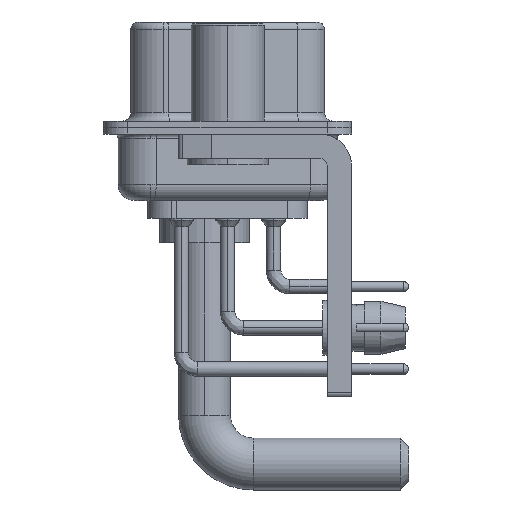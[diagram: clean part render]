
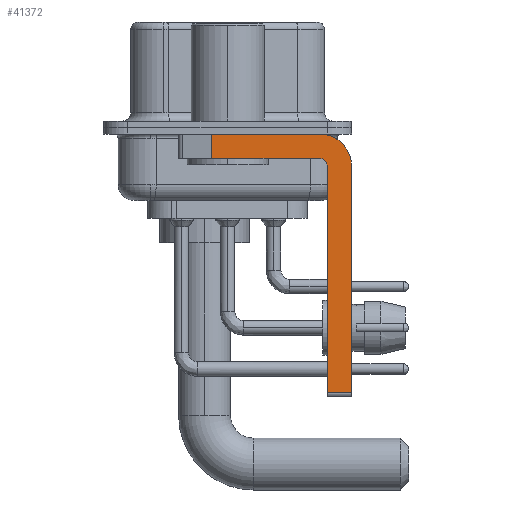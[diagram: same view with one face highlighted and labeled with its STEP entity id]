
A CAD part, left-side view. The second image highlights one B-rep face of the part: STEP entity #41372.
In plain terms, the highlighted planar face has unit normal (-1, 0, 0).
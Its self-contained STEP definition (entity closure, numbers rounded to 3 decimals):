
#185 = DIRECTION ( 'NONE',  ( 0., 0., -1. ) ) ;
#646 = CARTESIAN_POINT ( 'NONE',  ( -2.9, -7.65, -2.4 ) ) ;
#2032 = VERTEX_POINT ( 'NONE', #33714 ) ;
#2073 = LINE ( 'NONE', #14903, #31735 ) ;
#2317 = VECTOR ( 'NONE', #3384, 1000. ) ;
#2344 = EDGE_CURVE ( 'NONE', #15517, #5914, #19631, .T. ) ;
#2414 = ORIENTED_EDGE ( 'NONE', *, *, #25078, .F. ) ;
#2824 = VERTEX_POINT ( 'NONE', #13283 ) ;
#3009 = AXIS2_PLACEMENT_3D ( 'NONE', #11537, #37170, #8401 ) ;
#3141 = VERTEX_POINT ( 'NONE', #37407 ) ;
#3384 = DIRECTION ( 'NONE',  ( 0., -1., 0. ) ) ;
#4079 = DIRECTION ( 'NONE',  ( 0., 0., 1. ) ) ;
#4581 = ORIENTED_EDGE ( 'NONE', *, *, #2344, .F. ) ;
#4689 = DIRECTION ( 'NONE',  ( 0., 0., -1. ) ) ;
#5914 = VERTEX_POINT ( 'NONE', #8955 ) ;
#6447 = EDGE_CURVE ( 'NONE', #36493, #2032, #35358, .T. ) ;
#7075 = AXIS2_PLACEMENT_3D ( 'NONE', #7746, #20573, #36117 ) ;
#7746 = CARTESIAN_POINT ( 'NONE',  ( -2.9, -5.65, -2.4 ) ) ;
#7893 = AXIS2_PLACEMENT_3D ( 'NONE', #8662, #14952, #4689 ) ;
#8157 = EDGE_CURVE ( 'NONE', #36493, #9565, #31938, .T. ) ;
#8331 = ORIENTED_EDGE ( 'NONE', *, *, #39538, .T. ) ;
#8401 = DIRECTION ( 'NONE',  ( 0., 0., -1. ) ) ;
#8662 = CARTESIAN_POINT ( 'NONE',  ( -2.9, -5.65, -2.4 ) ) ;
#8955 = CARTESIAN_POINT ( 'NONE',  ( -2.9, -6.15, -2.4 ) ) ;
#9565 = VERTEX_POINT ( 'NONE', #18904 ) ;
#11042 = EDGE_CURVE ( 'NONE', #5914, #3141, #39941, .T. ) ;
#11537 = CARTESIAN_POINT ( 'NONE',  ( -2.9, -5.65, -2.4 ) ) ;
#12377 = VECTOR ( 'NONE', #185, 1000. ) ;
#13283 = CARTESIAN_POINT ( 'NONE',  ( -2.9, -7.65, -16.35 ) ) ;
#14903 = CARTESIAN_POINT ( 'NONE',  ( -2.9, -5.65, -1.9 ) ) ;
#14952 = DIRECTION ( 'NONE',  ( 1., 0., 0. ) ) ;
#15129 = PLANE ( 'NONE',  #3009 ) ;
#15517 = VERTEX_POINT ( 'NONE', #22314 ) ;
#16001 = CARTESIAN_POINT ( 'NONE',  ( -2.9, 0.978, -1.9 ) ) ;
#16626 = CIRCLE ( 'NONE', #7893, 2. ) ;
#16818 = ORIENTED_EDGE ( 'NONE', *, *, #6447, .F. ) ;
#18274 = FACE_OUTER_BOUND ( 'NONE', #23583, .T. ) ;
#18904 = CARTESIAN_POINT ( 'NONE',  ( -2.9, 0.978, -1.9 ) ) ;
#19631 = LINE ( 'NONE', #35584, #34057 ) ;
#20573 = DIRECTION ( 'NONE',  ( -1., 0., 0. ) ) ;
#21625 = DIRECTION ( 'NONE',  ( 0., 1., 0. ) ) ;
#21863 = LINE ( 'NONE', #32135, #12377 ) ;
#22314 = CARTESIAN_POINT ( 'NONE',  ( -2.9, -6.15, -16.35 ) ) ;
#22621 = ORIENTED_EDGE ( 'NONE', *, *, #8157, .T. ) ;
#23583 = EDGE_LOOP ( 'NONE', ( #16818, #22621, #32466, #31958, #4581, #8331, #2414, #29127 ) ) ;
#25078 = EDGE_CURVE ( 'NONE', #39558, #2824, #21863, .T. ) ;
#25511 = CARTESIAN_POINT ( 'NONE',  ( -2.9, 3., -0.4 ) ) ;
#28811 = DIRECTION ( 'NONE',  ( 0., 0., -1. ) ) ;
#29127 = ORIENTED_EDGE ( 'NONE', *, *, #33601, .F. ) ;
#31735 = VECTOR ( 'NONE', #21625, 1000. ) ;
#31938 = LINE ( 'NONE', #16001, #33811 ) ;
#31958 = ORIENTED_EDGE ( 'NONE', *, *, #11042, .F. ) ;
#32135 = CARTESIAN_POINT ( 'NONE',  ( -2.9, -7.65, -2.4 ) ) ;
#32466 = ORIENTED_EDGE ( 'NONE', *, *, #38532, .F. ) ;
#33601 = EDGE_CURVE ( 'NONE', #2032, #39558, #16626, .T. ) ;
#33714 = CARTESIAN_POINT ( 'NONE',  ( -2.9, -5.65, -0.4 ) ) ;
#33811 = VECTOR ( 'NONE', #28811, 1000. ) ;
#34057 = VECTOR ( 'NONE', #4079, 1000. ) ;
#34525 = DIRECTION ( 'NONE',  ( 0., -1., 0. ) ) ;
#35358 = LINE ( 'NONE', #25511, #39803 ) ;
#35389 = CARTESIAN_POINT ( 'NONE',  ( -2.9, 0.978, -0.4 ) ) ;
#35584 = CARTESIAN_POINT ( 'NONE',  ( -2.9, -6.15, -16.6 ) ) ;
#35725 = LINE ( 'NONE', #38260, #2317 ) ;
#36117 = DIRECTION ( 'NONE',  ( 0., 0., 1. ) ) ;
#36493 = VERTEX_POINT ( 'NONE', #35389 ) ;
#37170 = DIRECTION ( 'NONE',  ( 1., 0., 0. ) ) ;
#37407 = CARTESIAN_POINT ( 'NONE',  ( -2.9, -5.65, -1.9 ) ) ;
#38260 = CARTESIAN_POINT ( 'NONE',  ( -2.9, -5.65, -16.35 ) ) ;
#38532 = EDGE_CURVE ( 'NONE', #3141, #9565, #2073, .T. ) ;
#39538 = EDGE_CURVE ( 'NONE', #15517, #2824, #35725, .T. ) ;
#39558 = VERTEX_POINT ( 'NONE', #646 ) ;
#39803 = VECTOR ( 'NONE', #34525, 1000. ) ;
#39941 = CIRCLE ( 'NONE', #7075, 0.5 ) ;
#41372 = ADVANCED_FACE ( 'NONE', ( #18274 ), #15129, .F. ) ;
